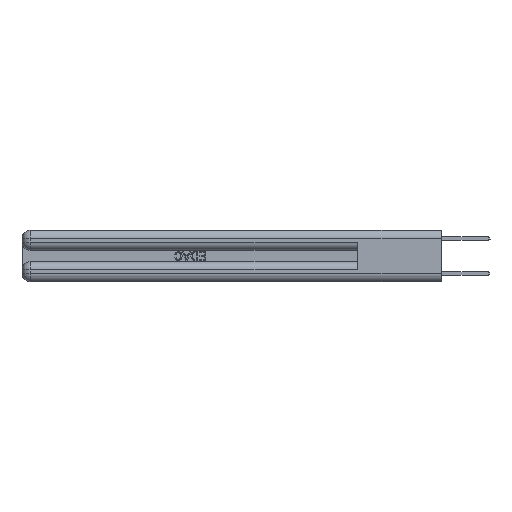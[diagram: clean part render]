
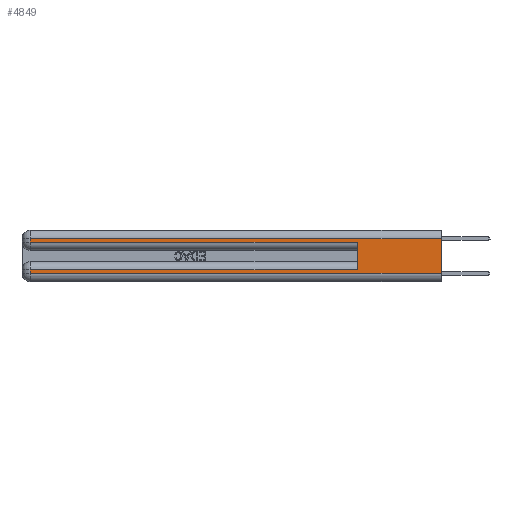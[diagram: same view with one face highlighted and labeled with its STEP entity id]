
A CAD part, left-side view. The second image highlights one B-rep face of the part: STEP entity #4849.
In plain terms, the highlighted planar face has unit normal (-1, 0, 0).
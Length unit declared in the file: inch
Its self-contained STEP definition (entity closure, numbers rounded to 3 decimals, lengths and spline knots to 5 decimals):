
#3 = DIRECTION ( 'NONE',  ( 0., 0., 1. ) ) ;
#185 = VERTEX_POINT ( 'NONE', #19613 ) ;
#208 = CARTESIAN_POINT ( 'NONE',  ( 0., 0.6, 0.145 ) ) ;
#2595 = LINE ( 'NONE', #208, #14944 ) ;
#3805 = PLANE ( 'NONE',  #29744 ) ;
#4557 = VERTEX_POINT ( 'NONE', #28247 ) ;
#4849 = ADVANCED_FACE ( 'NONE', ( #17920 ), #3805, .F. ) ;
#4895 = EDGE_CURVE ( 'NONE', #23254, #22741, #32793, .T. ) ;
#5992 = EDGE_CURVE ( 'NONE', #20149, #22741, #2595, .T. ) ;
#6878 = EDGE_CURVE ( 'NONE', #33949, #4557, #24203, .T. ) ;
#7126 = ORIENTED_EDGE ( 'NONE', *, *, #31956, .F. ) ;
#7812 = LINE ( 'NONE', #29700, #9841 ) ;
#7836 = CARTESIAN_POINT ( 'NONE',  ( 0., 2.94, 0.285 ) ) ;
#8398 = CARTESIAN_POINT ( 'NONE',  ( 0., 0., 0.285 ) ) ;
#8706 = VECTOR ( 'NONE', #32533, 39.37008 ) ;
#8911 = LINE ( 'NONE', #17351, #27116 ) ;
#9183 = ORIENTED_EDGE ( 'NONE', *, *, #6878, .T. ) ;
#9841 = VECTOR ( 'NONE', #24534, 39.37008 ) ;
#10733 = EDGE_CURVE ( 'NONE', #185, #23254, #28516, .T. ) ;
#11027 = CARTESIAN_POINT ( 'NONE',  ( 0., 0.6, 0.085 ) ) ;
#11774 = CARTESIAN_POINT ( 'NONE',  ( 0., 0., 0.37 ) ) ;
#12435 = VECTOR ( 'NONE', #20790, 39.37008 ) ;
#12446 = ORIENTED_EDGE ( 'NONE', *, *, #4895, .T. ) ;
#12618 = CARTESIAN_POINT ( 'NONE',  ( 0., 0., 0.06 ) ) ;
#13280 = CARTESIAN_POINT ( 'NONE',  ( 0., 0.6, 0.285 ) ) ;
#14083 = EDGE_CURVE ( 'NONE', #14533, #185, #8911, .T. ) ;
#14523 = LINE ( 'NONE', #30205, #8706 ) ;
#14533 = VERTEX_POINT ( 'NONE', #30192 ) ;
#14700 = ORIENTED_EDGE ( 'NONE', *, *, #10733, .T. ) ;
#14944 = VECTOR ( 'NONE', #3, 39.37008 ) ;
#15805 = VECTOR ( 'NONE', #24365, 39.37008 ) ;
#16213 = VERTEX_POINT ( 'NONE', #28914 ) ;
#17006 = EDGE_CURVE ( 'NONE', #20149, #16213, #14523, .T. ) ;
#17136 = VECTOR ( 'NONE', #25448, 39.37008 ) ;
#17351 = CARTESIAN_POINT ( 'NONE',  ( 0., 0., 0.31 ) ) ;
#17920 = FACE_OUTER_BOUND ( 'NONE', #19769, .T. ) ;
#18686 = LINE ( 'NONE', #28518, #31924 ) ;
#19606 = CARTESIAN_POINT ( 'NONE',  ( 0., 2.94, 0.06 ) ) ;
#19613 = CARTESIAN_POINT ( 'NONE',  ( 0., 2.94, 0.31 ) ) ;
#19769 = EDGE_LOOP ( 'NONE', ( #7126, #21606, #14700, #12446, #30384, #29238, #26062, #9183 ) ) ;
#20149 = VERTEX_POINT ( 'NONE', #11027 ) ;
#20274 = DIRECTION ( 'NONE',  ( 0., 1., 0. ) ) ;
#20532 = EDGE_CURVE ( 'NONE', #16213, #33949, #7812, .T. ) ;
#20790 = DIRECTION ( 'NONE',  ( 0., 0., -1. ) ) ;
#21606 = ORIENTED_EDGE ( 'NONE', *, *, #14083, .T. ) ;
#22741 = VERTEX_POINT ( 'NONE', #13280 ) ;
#23099 = DIRECTION ( 'NONE',  ( 0., 0., -1. ) ) ;
#23254 = VERTEX_POINT ( 'NONE', #7836 ) ;
#24203 = LINE ( 'NONE', #12618, #17136 ) ;
#24365 = DIRECTION ( 'NONE',  ( 0., -1., 0. ) ) ;
#24534 = DIRECTION ( 'NONE',  ( 0., 0., -1. ) ) ;
#25061 = DIRECTION ( 'NONE',  ( 1., 0., 0. ) ) ;
#25448 = DIRECTION ( 'NONE',  ( 0., -1., 0. ) ) ;
#26062 = ORIENTED_EDGE ( 'NONE', *, *, #20532, .T. ) ;
#26556 = CARTESIAN_POINT ( 'NONE',  ( 0., 2.94, 0.37 ) ) ;
#27116 = VECTOR ( 'NONE', #20274, 39.37008 ) ;
#28247 = CARTESIAN_POINT ( 'NONE',  ( 0., 0., 0.06 ) ) ;
#28516 = LINE ( 'NONE', #26556, #12435 ) ;
#28518 = CARTESIAN_POINT ( 'NONE',  ( 0., 0., 0.37 ) ) ;
#28914 = CARTESIAN_POINT ( 'NONE',  ( 0., 2.94, 0.085 ) ) ;
#29238 = ORIENTED_EDGE ( 'NONE', *, *, #17006, .T. ) ;
#29700 = CARTESIAN_POINT ( 'NONE',  ( 0., 2.94, 0.37 ) ) ;
#29744 = AXIS2_PLACEMENT_3D ( 'NONE', #11774, #25061, #23099 ) ;
#30192 = CARTESIAN_POINT ( 'NONE',  ( 0., 0., 0.31 ) ) ;
#30205 = CARTESIAN_POINT ( 'NONE',  ( 0., 0., 0.085 ) ) ;
#30384 = ORIENTED_EDGE ( 'NONE', *, *, #5992, .F. ) ;
#31090 = DIRECTION ( 'NONE',  ( 0., 0., -1. ) ) ;
#31924 = VECTOR ( 'NONE', #31090, 39.37008 ) ;
#31956 = EDGE_CURVE ( 'NONE', #14533, #4557, #18686, .T. ) ;
#32533 = DIRECTION ( 'NONE',  ( 0., 1., 0. ) ) ;
#32793 = LINE ( 'NONE', #8398, #15805 ) ;
#33949 = VERTEX_POINT ( 'NONE', #19606 ) ;
